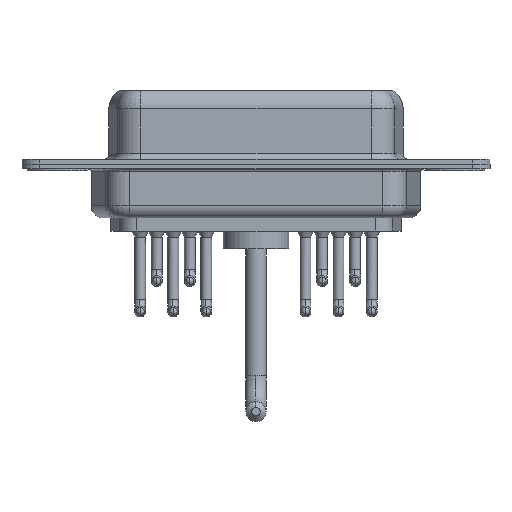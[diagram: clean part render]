
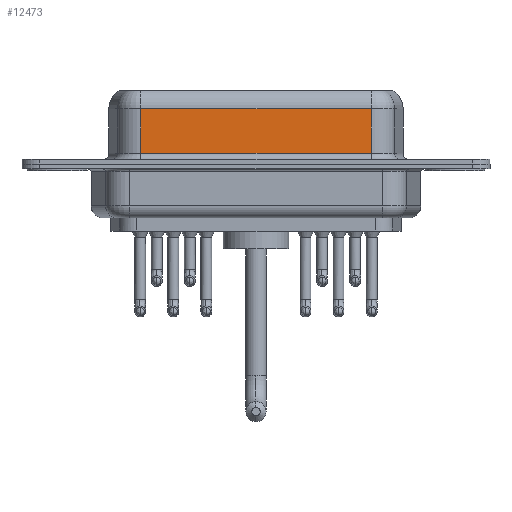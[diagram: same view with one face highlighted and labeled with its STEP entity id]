
A CAD part, front view. The second image highlights one B-rep face of the part: STEP entity #12473.
In plain terms, the highlighted planar face has unit normal (0, -1, 0).
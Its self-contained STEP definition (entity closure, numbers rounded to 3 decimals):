
#133 = VECTOR ( 'NONE', #10116, 1000. ) ;
#414 = EDGE_CURVE ( 'NONE', #16390, #12441, #2606, .T. ) ;
#415 = VERTEX_POINT ( 'NONE', #10467 ) ;
#1021 = VECTOR ( 'NONE', #6424, 1000. ) ;
#2606 = LINE ( 'NONE', #14383, #7970 ) ;
#3168 = EDGE_LOOP ( 'NONE', ( #12324, #13391, #9383, #5376 ) ) ;
#3250 = DIRECTION ( 'NONE',  ( 0., 1., 0. ) ) ;
#4454 = FACE_OUTER_BOUND ( 'NONE', #3168, .T. ) ;
#5376 = ORIENTED_EDGE ( 'NONE', *, *, #13112, .T. ) ;
#6204 = EDGE_CURVE ( 'NONE', #16390, #415, #7796, .T. ) ;
#6424 = DIRECTION ( 'NONE',  ( -1., 0., 0. ) ) ;
#6440 = CARTESIAN_POINT ( 'NONE',  ( 7.013, -3.95, 6.4 ) ) ;
#7231 = VERTEX_POINT ( 'NONE', #12249 ) ;
#7796 = LINE ( 'NONE', #16768, #1021 ) ;
#7820 = DIRECTION ( 'NONE',  ( 0., 0., -1. ) ) ;
#7970 = VECTOR ( 'NONE', #7820, 1000. ) ;
#8786 = DIRECTION ( 'NONE',  ( 1., 0., 0. ) ) ;
#9014 = AXIS2_PLACEMENT_3D ( 'NONE', #13758, #3250, #12388 ) ;
#9383 = ORIENTED_EDGE ( 'NONE', *, *, #10336, .T. ) ;
#10116 = DIRECTION ( 'NONE',  ( 0., 0., -1. ) ) ;
#10336 = EDGE_CURVE ( 'NONE', #415, #7231, #12673, .T. ) ;
#10467 = CARTESIAN_POINT ( 'NONE',  ( 7.013, -3.95, 4.65 ) ) ;
#11229 = CARTESIAN_POINT ( 'NONE',  ( 26.287, -3.95, 4.65 ) ) ;
#11354 = CARTESIAN_POINT ( 'NONE',  ( 26.287, -3.95, 0.9 ) ) ;
#12227 = PLANE ( 'NONE',  #9014 ) ;
#12249 = CARTESIAN_POINT ( 'NONE',  ( 7.013, -3.95, 0.9 ) ) ;
#12324 = ORIENTED_EDGE ( 'NONE', *, *, #414, .F. ) ;
#12388 = DIRECTION ( 'NONE',  ( 0., 0., 1. ) ) ;
#12441 = VERTEX_POINT ( 'NONE', #12472 ) ;
#12458 = LINE ( 'NONE', #11354, #12579 ) ;
#12472 = CARTESIAN_POINT ( 'NONE',  ( 26.287, -3.95, 0.9 ) ) ;
#12473 = ADVANCED_FACE ( 'NONE', ( #4454 ), #12227, .F. ) ;
#12579 = VECTOR ( 'NONE', #8786, 1000. ) ;
#12673 = LINE ( 'NONE', #6440, #133 ) ;
#13112 = EDGE_CURVE ( 'NONE', #7231, #12441, #12458, .T. ) ;
#13391 = ORIENTED_EDGE ( 'NONE', *, *, #6204, .T. ) ;
#13758 = CARTESIAN_POINT ( 'NONE',  ( 26.287, -3.95, 6.4 ) ) ;
#14383 = CARTESIAN_POINT ( 'NONE',  ( 26.287, -3.95, 6.4 ) ) ;
#16390 = VERTEX_POINT ( 'NONE', #11229 ) ;
#16768 = CARTESIAN_POINT ( 'NONE',  ( 26.287, -3.95, 4.65 ) ) ;
